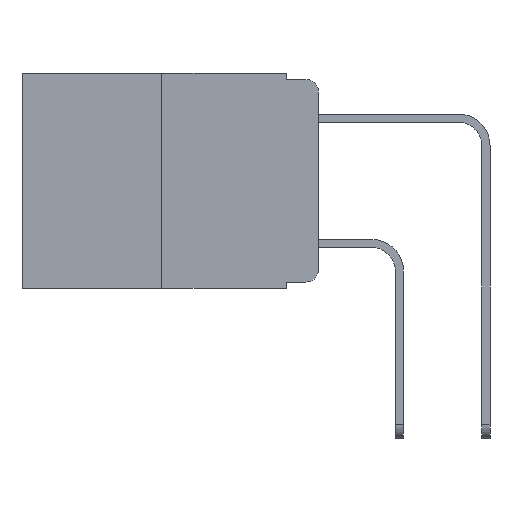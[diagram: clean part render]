
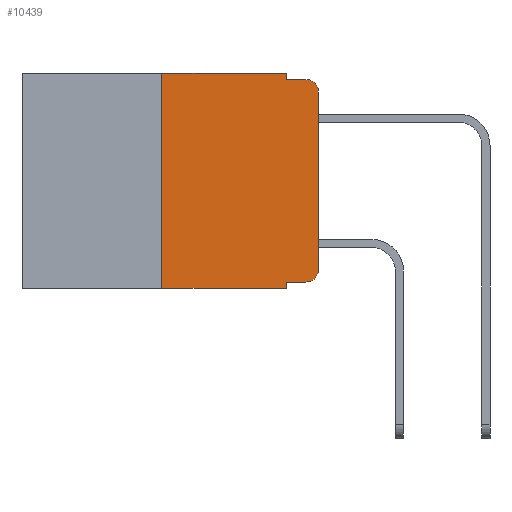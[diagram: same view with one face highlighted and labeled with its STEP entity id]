
A CAD part, left-side view. The second image highlights one B-rep face of the part: STEP entity #10439.
In plain terms, the highlighted planar face has unit normal (-1, 0, 0).
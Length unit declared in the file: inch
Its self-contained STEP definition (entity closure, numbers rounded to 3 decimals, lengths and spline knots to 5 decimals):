
#68 = AXIS2_PLACEMENT_3D ( 'NONE', #4127, #6076, #9090 ) ;
#193 = DIRECTION ( 'NONE',  ( 0., -1., 0. ) ) ;
#225 = VERTEX_POINT ( 'NONE', #12829 ) ;
#332 = CARTESIAN_POINT ( 'NONE',  ( 0., 0.02, -0.333 ) ) ;
#406 = EDGE_CURVE ( 'NONE', #225, #7532, #690, .T. ) ;
#690 = CIRCLE ( 'NONE', #68, 0.02 ) ;
#997 = CIRCLE ( 'NONE', #4367, 0.02 ) ;
#1627 = VECTOR ( 'NONE', #193, 39.37008 ) ;
#1632 = VERTEX_POINT ( 'NONE', #4132 ) ;
#1739 = EDGE_CURVE ( 'NONE', #12824, #10692, #1901, .T. ) ;
#1901 = LINE ( 'NONE', #9529, #7544 ) ;
#1910 = EDGE_CURVE ( 'NONE', #5416, #225, #8033, .T. ) ;
#1965 = ORIENTED_EDGE ( 'NONE', *, *, #10604, .F. ) ;
#2210 = ORIENTED_EDGE ( 'NONE', *, *, #7152, .T. ) ;
#2429 = CARTESIAN_POINT ( 'NONE',  ( 0., 0.25, 0. ) ) ;
#2572 = ORIENTED_EDGE ( 'NONE', *, *, #3567, .T. ) ;
#2791 = ORIENTED_EDGE ( 'NONE', *, *, #7867, .T. ) ;
#2873 = CARTESIAN_POINT ( 'NONE',  ( 0., 0.051, 0. ) ) ;
#2941 = ORIENTED_EDGE ( 'NONE', *, *, #406, .T. ) ;
#3107 = VERTEX_POINT ( 'NONE', #7499 ) ;
#3130 = DIRECTION ( 'NONE',  ( 0., 0., 1. ) ) ;
#3486 = CARTESIAN_POINT ( 'NONE',  ( 0., 0.02, -0.313 ) ) ;
#3567 = EDGE_CURVE ( 'NONE', #3107, #1632, #7497, .T. ) ;
#3629 = ORIENTED_EDGE ( 'NONE', *, *, #8562, .F. ) ;
#3922 = CARTESIAN_POINT ( 'NONE',  ( 0., 0.473, 0. ) ) ;
#4127 = CARTESIAN_POINT ( 'NONE',  ( 0., 0.02, -0.03 ) ) ;
#4132 = CARTESIAN_POINT ( 'NONE',  ( 0., 0.051, -0.343 ) ) ;
#4157 = LINE ( 'NONE', #10797, #1627 ) ;
#4354 = LINE ( 'NONE', #10506, #12219 ) ;
#4367 = AXIS2_PLACEMENT_3D ( 'NONE', #3486, #10751, #4544 ) ;
#4538 = VECTOR ( 'NONE', #3130, 39.37008 ) ;
#4544 = DIRECTION ( 'NONE',  ( 0., 0., -1. ) ) ;
#4960 = DIRECTION ( 'NONE',  ( 1., 0., 0. ) ) ;
#5323 = DIRECTION ( 'NONE',  ( 0., 0., -1. ) ) ;
#5416 = VERTEX_POINT ( 'NONE', #8134 ) ;
#5618 = AXIS2_PLACEMENT_3D ( 'NONE', #3922, #4960, #12149 ) ;
#5825 = VECTOR ( 'NONE', #8787, 39.37008 ) ;
#6076 = DIRECTION ( 'NONE',  ( -1., 0., 0. ) ) ;
#6110 = CARTESIAN_POINT ( 'NONE',  ( 0., 0.02, -0.01 ) ) ;
#6364 = DIRECTION ( 'NONE',  ( 0., -1., 0. ) ) ;
#6498 = ORIENTED_EDGE ( 'NONE', *, *, #1739, .F. ) ;
#6928 = ORIENTED_EDGE ( 'NONE', *, *, #11926, .F. ) ;
#7152 = EDGE_CURVE ( 'NONE', #8981, #5416, #997, .T. ) ;
#7497 = LINE ( 'NONE', #12438, #9929 ) ;
#7499 = CARTESIAN_POINT ( 'NONE',  ( 0., 0.25, -0.343 ) ) ;
#7532 = VERTEX_POINT ( 'NONE', #6110 ) ;
#7544 = VECTOR ( 'NONE', #6364, 39.37008 ) ;
#7719 = CARTESIAN_POINT ( 'NONE',  ( 0., 0., 0. ) ) ;
#7820 = CARTESIAN_POINT ( 'NONE',  ( 0., 0.051, -0.01 ) ) ;
#7867 = EDGE_CURVE ( 'NONE', #10762, #8981, #8639, .T. ) ;
#8033 = LINE ( 'NONE', #7719, #8693 ) ;
#8134 = CARTESIAN_POINT ( 'NONE',  ( 0., 0., -0.313 ) ) ;
#8157 = EDGE_LOOP ( 'NONE', ( #9311, #2941, #6928, #8323, #6498, #1965, #2572, #3629, #2791, #2210 ) ) ;
#8323 = ORIENTED_EDGE ( 'NONE', *, *, #11259, .F. ) ;
#8377 = VERTEX_POINT ( 'NONE', #7820 ) ;
#8562 = EDGE_CURVE ( 'NONE', #10762, #1632, #13434, .T. ) ;
#8639 = LINE ( 'NONE', #12772, #5825 ) ;
#8693 = VECTOR ( 'NONE', #11745, 39.37008 ) ;
#8787 = DIRECTION ( 'NONE',  ( 0., -1., 0. ) ) ;
#8981 = VERTEX_POINT ( 'NONE', #332 ) ;
#9090 = DIRECTION ( 'NONE',  ( 0., 0., -1. ) ) ;
#9311 = ORIENTED_EDGE ( 'NONE', *, *, #1910, .T. ) ;
#9529 = CARTESIAN_POINT ( 'NONE',  ( 0., 0.473, 0. ) ) ;
#9929 = VECTOR ( 'NONE', #11455, 39.37008 ) ;
#10170 = PLANE ( 'NONE',  #5618 ) ;
#10419 = CARTESIAN_POINT ( 'NONE',  ( 0., 0.25, 0. ) ) ;
#10439 = ADVANCED_FACE ( 'NONE', ( #12244 ), #10170, .F. ) ;
#10506 = CARTESIAN_POINT ( 'NONE',  ( 0., 0.051, 0. ) ) ;
#10604 = EDGE_CURVE ( 'NONE', #3107, #12824, #10702, .T. ) ;
#10682 = CARTESIAN_POINT ( 'NONE',  ( 0., 0.051, -0.333 ) ) ;
#10692 = VERTEX_POINT ( 'NONE', #12541 ) ;
#10702 = LINE ( 'NONE', #10419, #4538 ) ;
#10751 = DIRECTION ( 'NONE',  ( -1., 0., 0. ) ) ;
#10762 = VERTEX_POINT ( 'NONE', #10682 ) ;
#10797 = CARTESIAN_POINT ( 'NONE',  ( 0., 0.051, -0.01 ) ) ;
#10833 = VECTOR ( 'NONE', #11185, 39.37008 ) ;
#11185 = DIRECTION ( 'NONE',  ( 0., 0., -1. ) ) ;
#11259 = EDGE_CURVE ( 'NONE', #10692, #8377, #4354, .T. ) ;
#11455 = DIRECTION ( 'NONE',  ( 0., -1., 0. ) ) ;
#11745 = DIRECTION ( 'NONE',  ( 0., 0., 1. ) ) ;
#11926 = EDGE_CURVE ( 'NONE', #8377, #7532, #4157, .T. ) ;
#12149 = DIRECTION ( 'NONE',  ( 0., 0., -1. ) ) ;
#12219 = VECTOR ( 'NONE', #5323, 39.37008 ) ;
#12244 = FACE_OUTER_BOUND ( 'NONE', #8157, .T. ) ;
#12438 = CARTESIAN_POINT ( 'NONE',  ( 0., 0.473, -0.343 ) ) ;
#12541 = CARTESIAN_POINT ( 'NONE',  ( 0., 0.051, 0. ) ) ;
#12772 = CARTESIAN_POINT ( 'NONE',  ( 0., 0.051, -0.333 ) ) ;
#12824 = VERTEX_POINT ( 'NONE', #2429 ) ;
#12829 = CARTESIAN_POINT ( 'NONE',  ( 0., 0., -0.03 ) ) ;
#13434 = LINE ( 'NONE', #2873, #10833 ) ;
